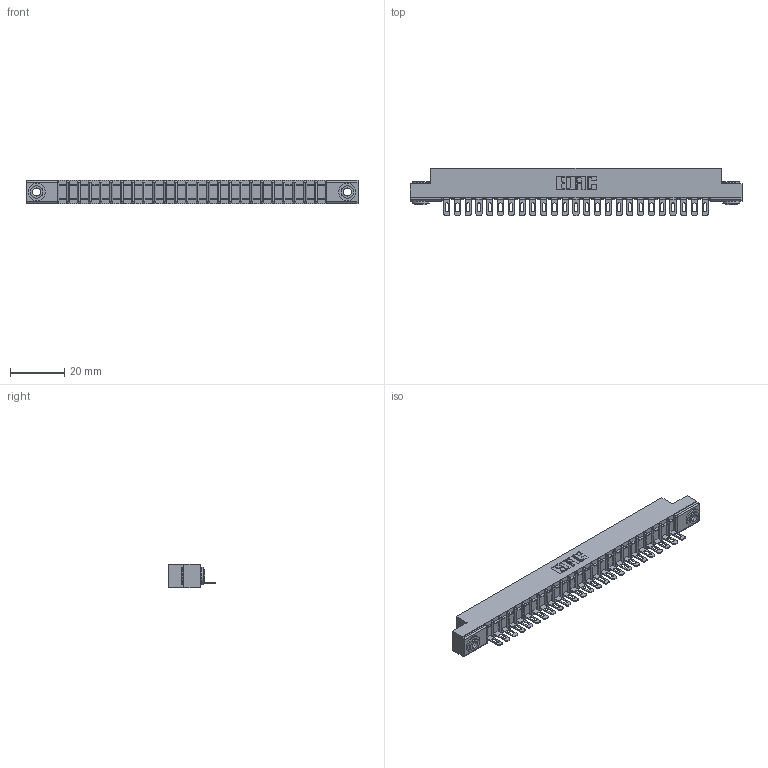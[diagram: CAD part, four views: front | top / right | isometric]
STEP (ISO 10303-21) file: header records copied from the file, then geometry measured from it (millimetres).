
FILE_DESCRIPTION (( 'STEP AP203' ), '1' );
FILE_NAME ('307-025-401-103.STEP', '2020-09-27T13:32:30', ( '' ), ( '' ), 'SwSTEP 2.0', 'SolidWorks 2020', '' );
FILE_SCHEMA (( 'CONFIG_CONTROL_DESIGN' ));
Length unit declared in the file: inch
Products named in the file (4): 307-290-002_501; 307 Part_.156 Dia Mounting Holes; 345-250-002_345-250-002-102; 307-025-401-103
Assembly tree (28 placements, depth 2):
  307-025-401-103
    307 Part_.156 Dia Mounting Holes
    307-290-002_501  x25
    345-250-002_345-250-002-102  x2
Bounding box: 122.07 x 17.42 x 8.71 mm (x, y, z)
Volume: 8083.6 mm3; surface area: 15281.8 mm2
Topology: 28 solids, 28 shells, 2096 faces, 6385 edges, 4182 vertices
Faces by surface type: plane 1194, cylinder 842, sphere 52, cone 8
Entity records: 25387 total; most frequent: CARTESIAN_POINT 4257, ORIENTED_EDGE 4238, DIRECTION 4163, EDGE_CURVE 2119, VECTOR 1603, LINE 1603, VERTEX_POINT 1374, AXIS2_PLACEMENT_3D 1280
